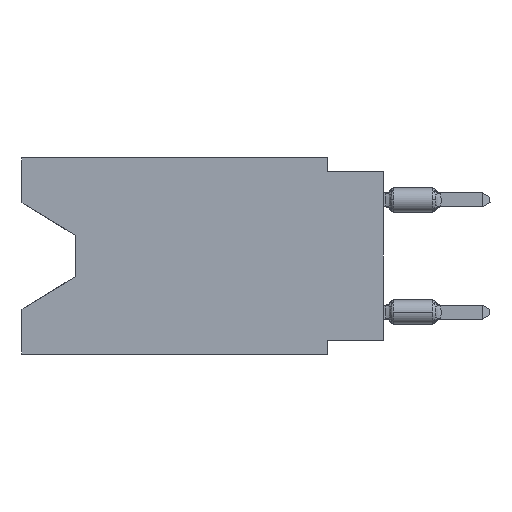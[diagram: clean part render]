
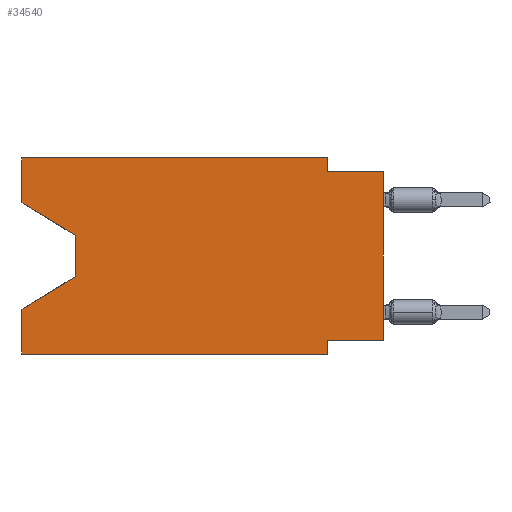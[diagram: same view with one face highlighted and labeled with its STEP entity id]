
A CAD part, left-side view. The second image highlights one B-rep face of the part: STEP entity #34540.
In plain terms, the highlighted planar face has unit normal (-1, 0, 0).
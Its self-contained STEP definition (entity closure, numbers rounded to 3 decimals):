
#988 = DIRECTION ( 'NONE',  ( 0., 1., 0. ) ) ;
#1074 = VECTOR ( 'NONE', #988, 1000. ) ;
#1217 = VECTOR ( 'NONE', #22092, 1000. ) ;
#1226 = CARTESIAN_POINT ( 'NONE',  ( 0., 13.97, -5.385 ) ) ;
#2255 = ORIENTED_EDGE ( 'NONE', *, *, #32912, .T. ) ;
#2531 = CARTESIAN_POINT ( 'NONE',  ( 0., 2.54, 0. ) ) ;
#2845 = VERTEX_POINT ( 'NONE', #39861 ) ;
#3203 = CARTESIAN_POINT ( 'NONE',  ( 0., 16.383, -8.89 ) ) ;
#4296 = DIRECTION ( 'NONE',  ( 0., 0., 1. ) ) ;
#4607 = CARTESIAN_POINT ( 'NONE',  ( 0., 16.383, -8.89 ) ) ;
#4623 = PLANE ( 'NONE',  #11513 ) ;
#4874 = DIRECTION ( 'NONE',  ( 0., 0., -1. ) ) ;
#5151 = VECTOR ( 'NONE', #43215, 1000. ) ;
#5189 = VECTOR ( 'NONE', #23791, 1000. ) ;
#5631 = EDGE_CURVE ( 'NONE', #29809, #15404, #31830, .T. ) ;
#8021 = LINE ( 'NONE', #38067, #31421 ) ;
#9705 = VERTEX_POINT ( 'NONE', #48009 ) ;
#11109 = LINE ( 'NONE', #3203, #41030 ) ;
#11332 = CARTESIAN_POINT ( 'NONE',  ( 0., 2.54, -8.255 ) ) ;
#11428 = VERTEX_POINT ( 'NONE', #43989 ) ;
#11513 = AXIS2_PLACEMENT_3D ( 'NONE', #27776, #27299, #4874 ) ;
#13081 = ORIENTED_EDGE ( 'NONE', *, *, #28311, .F. ) ;
#13336 = CARTESIAN_POINT ( 'NONE',  ( 0., 16.383, 0. ) ) ;
#13573 = CARTESIAN_POINT ( 'NONE',  ( 0., 2.54, -0.635 ) ) ;
#13907 = ORIENTED_EDGE ( 'NONE', *, *, #5631, .F. ) ;
#14667 = VECTOR ( 'NONE', #41095, 1000. ) ;
#15404 = VERTEX_POINT ( 'NONE', #42497 ) ;
#15788 = DIRECTION ( 'NONE',  ( 0., 0.855, -0.519 ) ) ;
#15797 = ORIENTED_EDGE ( 'NONE', *, *, #33255, .F. ) ;
#15839 = LINE ( 'NONE', #41224, #27193 ) ;
#16020 = LINE ( 'NONE', #1226, #34908 ) ;
#17627 = CARTESIAN_POINT ( 'NONE',  ( 0., 16.383, -2.038 ) ) ;
#17847 = EDGE_CURVE ( 'NONE', #19687, #2845, #11109, .T. ) ;
#18172 = EDGE_CURVE ( 'NONE', #25359, #29800, #21870, .T. ) ;
#19687 = VERTEX_POINT ( 'NONE', #4607 ) ;
#19726 = LINE ( 'NONE', #46568, #1074 ) ;
#20086 = LINE ( 'NONE', #38343, #5189 ) ;
#20134 = FACE_OUTER_BOUND ( 'NONE', #38721, .T. ) ;
#20307 = LINE ( 'NONE', #28189, #5151 ) ;
#21870 = LINE ( 'NONE', #40859, #14667 ) ;
#21929 = DIRECTION ( 'NONE',  ( 0., -1., 0. ) ) ;
#22092 = DIRECTION ( 'NONE',  ( 0., 0., -1. ) ) ;
#22297 = VECTOR ( 'NONE', #42193, 1000. ) ;
#22593 = CARTESIAN_POINT ( 'NONE',  ( 0., 13.97, -3.505 ) ) ;
#22943 = VECTOR ( 'NONE', #43163, 1000. ) ;
#23780 = ORIENTED_EDGE ( 'NONE', *, *, #46248, .F. ) ;
#23791 = DIRECTION ( 'NONE',  ( 0., 0., -1. ) ) ;
#24157 = CARTESIAN_POINT ( 'NONE',  ( 0., 13.97, -5.385 ) ) ;
#25359 = VERTEX_POINT ( 'NONE', #41319 ) ;
#26234 = VERTEX_POINT ( 'NONE', #11332 ) ;
#26699 = DIRECTION ( 'NONE',  ( 0., 0., 1. ) ) ;
#27193 = VECTOR ( 'NONE', #26699, 1000. ) ;
#27299 = DIRECTION ( 'NONE',  ( 1., 0., 0. ) ) ;
#27776 = CARTESIAN_POINT ( 'NONE',  ( 0., 16.383, 0. ) ) ;
#28189 = CARTESIAN_POINT ( 'NONE',  ( 0., 16.383, 0. ) ) ;
#28311 = EDGE_CURVE ( 'NONE', #19687, #11428, #8021, .T. ) ;
#28625 = VERTEX_POINT ( 'NONE', #24157 ) ;
#29470 = DIRECTION ( 'NONE',  ( 0., -0.855, -0.519 ) ) ;
#29800 = VERTEX_POINT ( 'NONE', #13336 ) ;
#29809 = VERTEX_POINT ( 'NONE', #13573 ) ;
#30167 = ORIENTED_EDGE ( 'NONE', *, *, #39758, .F. ) ;
#31421 = VECTOR ( 'NONE', #4296, 1000. ) ;
#31462 = ORIENTED_EDGE ( 'NONE', *, *, #40104, .T. ) ;
#31740 = VERTEX_POINT ( 'NONE', #34909 ) ;
#31830 = LINE ( 'NONE', #32074, #22943 ) ;
#32071 = CARTESIAN_POINT ( 'NONE',  ( 0., 2.54, -8.89 ) ) ;
#32074 = CARTESIAN_POINT ( 'NONE',  ( 0., 0., -0.635 ) ) ;
#32912 = EDGE_CURVE ( 'NONE', #25359, #31740, #40541, .T. ) ;
#33255 = EDGE_CURVE ( 'NONE', #29800, #33409, #20307, .T. ) ;
#33409 = VERTEX_POINT ( 'NONE', #2531 ) ;
#33531 = EDGE_CURVE ( 'NONE', #9705, #15404, #15839, .T. ) ;
#34540 = ADVANCED_FACE ( 'NONE', ( #20134 ), #4623, .F. ) ;
#34908 = VECTOR ( 'NONE', #15788, 1000. ) ;
#34909 = CARTESIAN_POINT ( 'NONE',  ( 0., 13.97, -3.505 ) ) ;
#36091 = EDGE_CURVE ( 'NONE', #33409, #29809, #20086, .T. ) ;
#36890 = LINE ( 'NONE', #22593, #1217 ) ;
#38054 = ORIENTED_EDGE ( 'NONE', *, *, #48081, .T. ) ;
#38067 = CARTESIAN_POINT ( 'NONE',  ( 0., 16.383, 0. ) ) ;
#38343 = CARTESIAN_POINT ( 'NONE',  ( 0., 2.54, 0. ) ) ;
#38721 = EDGE_LOOP ( 'NONE', ( #2255, #38054, #31462, #13081, #39456, #30167, #23780, #43452, #13907, #48364, #15797, #46321 ) ) ;
#39456 = ORIENTED_EDGE ( 'NONE', *, *, #17847, .T. ) ;
#39475 = LINE ( 'NONE', #32071, #22297 ) ;
#39758 = EDGE_CURVE ( 'NONE', #26234, #2845, #39475, .T. ) ;
#39861 = CARTESIAN_POINT ( 'NONE',  ( 0., 2.54, -8.89 ) ) ;
#40104 = EDGE_CURVE ( 'NONE', #28625, #11428, #16020, .T. ) ;
#40541 = LINE ( 'NONE', #17627, #47919 ) ;
#40859 = CARTESIAN_POINT ( 'NONE',  ( 0., 16.383, 0. ) ) ;
#41030 = VECTOR ( 'NONE', #21929, 1000. ) ;
#41095 = DIRECTION ( 'NONE',  ( 0., 0., 1. ) ) ;
#41224 = CARTESIAN_POINT ( 'NONE',  ( 0., 0., 0. ) ) ;
#41319 = CARTESIAN_POINT ( 'NONE',  ( 0., 16.383, -2.038 ) ) ;
#42193 = DIRECTION ( 'NONE',  ( 0., 0., -1. ) ) ;
#42497 = CARTESIAN_POINT ( 'NONE',  ( 0., 0., -0.635 ) ) ;
#43163 = DIRECTION ( 'NONE',  ( 0., -1., 0. ) ) ;
#43215 = DIRECTION ( 'NONE',  ( 0., -1., 0. ) ) ;
#43452 = ORIENTED_EDGE ( 'NONE', *, *, #33531, .T. ) ;
#43989 = CARTESIAN_POINT ( 'NONE',  ( 0., 16.383, -6.852 ) ) ;
#46248 = EDGE_CURVE ( 'NONE', #9705, #26234, #19726, .T. ) ;
#46321 = ORIENTED_EDGE ( 'NONE', *, *, #18172, .F. ) ;
#46568 = CARTESIAN_POINT ( 'NONE',  ( 0., 0., -8.255 ) ) ;
#47919 = VECTOR ( 'NONE', #29470, 1000. ) ;
#48009 = CARTESIAN_POINT ( 'NONE',  ( 0., 0., -8.255 ) ) ;
#48081 = EDGE_CURVE ( 'NONE', #31740, #28625, #36890, .T. ) ;
#48364 = ORIENTED_EDGE ( 'NONE', *, *, #36091, .F. ) ;
